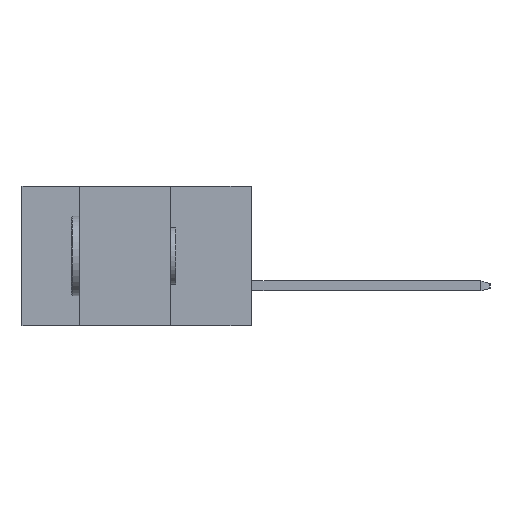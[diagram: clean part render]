
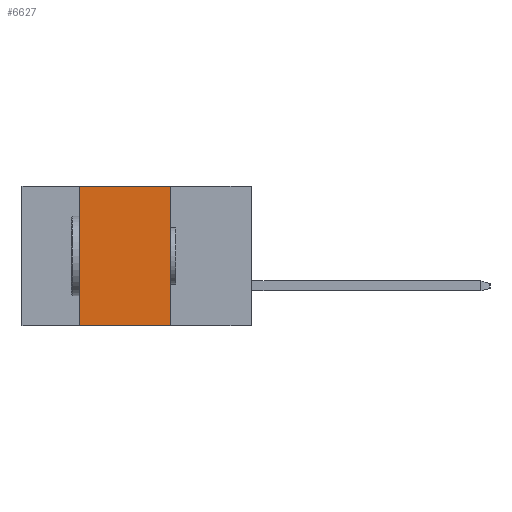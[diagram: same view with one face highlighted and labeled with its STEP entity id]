
A CAD part, left-side view. The second image highlights one B-rep face of the part: STEP entity #6627.
In plain terms, the highlighted planar face has unit normal (-1, 0, 0).
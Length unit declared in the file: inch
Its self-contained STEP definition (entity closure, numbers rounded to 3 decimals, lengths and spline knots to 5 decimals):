
#420 = LINE ( 'NONE', #9613, #8275 ) ;
#633 = LINE ( 'NONE', #7453, #10896 ) ;
#965 = LINE ( 'NONE', #8620, #2512 ) ;
#1543 = EDGE_LOOP ( 'NONE', ( #9369, #2575, #11586, #9462 ) ) ;
#2247 = PLANE ( 'NONE',  #10868 ) ;
#2369 = DIRECTION ( 'NONE',  ( 1., 0., 0. ) ) ;
#2394 = EDGE_CURVE ( 'NONE', #12500, #12408, #965, .T. ) ;
#2512 = VECTOR ( 'NONE', #2900, 39.37008 ) ;
#2575 = ORIENTED_EDGE ( 'NONE', *, *, #4997, .F. ) ;
#2900 = DIRECTION ( 'NONE',  ( 0., 0., 1. ) ) ;
#3209 = DIRECTION ( 'NONE',  ( 0., 0., -1. ) ) ;
#3729 = DIRECTION ( 'NONE',  ( 0., -1., 0. ) ) ;
#4239 = EDGE_CURVE ( 'NONE', #12500, #4412, #633, .T. ) ;
#4412 = VERTEX_POINT ( 'NONE', #6433 ) ;
#4997 = EDGE_CURVE ( 'NONE', #12408, #8928, #12569, .T. ) ;
#5324 = CARTESIAN_POINT ( 'NONE',  ( 0., 0.54, 0. ) ) ;
#6095 = CARTESIAN_POINT ( 'NONE',  ( 0., 0.72, 0. ) ) ;
#6139 = CARTESIAN_POINT ( 'NONE',  ( 0., 0.54, -0.437 ) ) ;
#6433 = CARTESIAN_POINT ( 'NONE',  ( 0., 0.254, -0.437 ) ) ;
#6627 = ADVANCED_FACE ( 'NONE', ( #11165 ), #2247, .F. ) ;
#6984 = VECTOR ( 'NONE', #10648, 39.37008 ) ;
#7453 = CARTESIAN_POINT ( 'NONE',  ( 0., 0.72, -0.437 ) ) ;
#8275 = VECTOR ( 'NONE', #10632, 39.37008 ) ;
#8620 = CARTESIAN_POINT ( 'NONE',  ( 0., 0.54, -0.437 ) ) ;
#8826 = EDGE_CURVE ( 'NONE', #8928, #4412, #420, .T. ) ;
#8928 = VERTEX_POINT ( 'NONE', #10442 ) ;
#9369 = ORIENTED_EDGE ( 'NONE', *, *, #8826, .F. ) ;
#9462 = ORIENTED_EDGE ( 'NONE', *, *, #4239, .T. ) ;
#9613 = CARTESIAN_POINT ( 'NONE',  ( 0., 0.254, -0.437 ) ) ;
#10442 = CARTESIAN_POINT ( 'NONE',  ( 0., 0.254, 0. ) ) ;
#10632 = DIRECTION ( 'NONE',  ( 0., 0., -1. ) ) ;
#10648 = DIRECTION ( 'NONE',  ( 0., -1., 0. ) ) ;
#10868 = AXIS2_PLACEMENT_3D ( 'NONE', #6095, #2369, #3209 ) ;
#10896 = VECTOR ( 'NONE', #3729, 39.37008 ) ;
#11165 = FACE_OUTER_BOUND ( 'NONE', #1543, .T. ) ;
#11586 = ORIENTED_EDGE ( 'NONE', *, *, #2394, .F. ) ;
#11867 = CARTESIAN_POINT ( 'NONE',  ( 0., 0.72, 0. ) ) ;
#12408 = VERTEX_POINT ( 'NONE', #5324 ) ;
#12500 = VERTEX_POINT ( 'NONE', #6139 ) ;
#12569 = LINE ( 'NONE', #11867, #6984 ) ;
